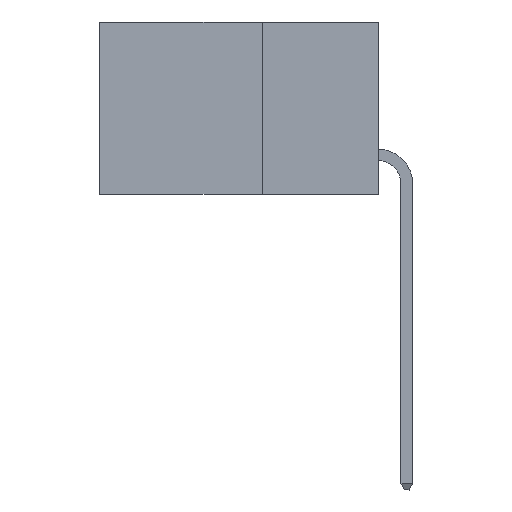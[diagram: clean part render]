
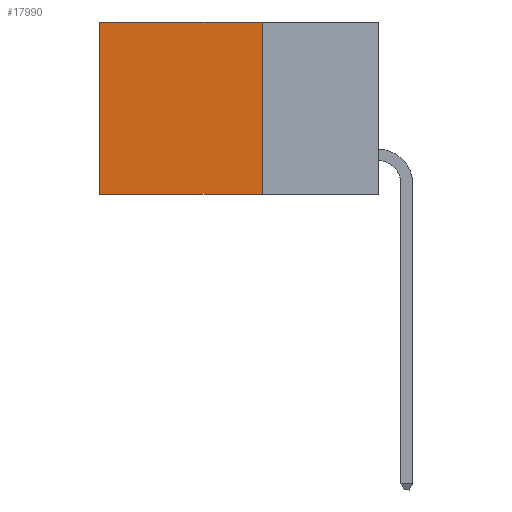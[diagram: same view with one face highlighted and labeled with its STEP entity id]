
A CAD part, left-side view. The second image highlights one B-rep face of the part: STEP entity #17990.
In plain terms, the highlighted planar face has unit normal (-1, 0, 0).
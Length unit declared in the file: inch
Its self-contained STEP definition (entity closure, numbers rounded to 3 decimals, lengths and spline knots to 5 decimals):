
#1260 = DIRECTION ( 'NONE',  ( 1., 0., 0. ) ) ;
#1993 = CARTESIAN_POINT ( 'NONE',  ( 0.298, 0.25, -0.37 ) ) ;
#3999 = LINE ( 'NONE', #11237, #13627 ) ;
#4737 = CARTESIAN_POINT ( 'NONE',  ( 0.298, 0.25, 0. ) ) ;
#4782 = VERTEX_POINT ( 'NONE', #7912 ) ;
#6050 = ORIENTED_EDGE ( 'NONE', *, *, #15029, .F. ) ;
#7912 = CARTESIAN_POINT ( 'NONE',  ( 0.298, 0.6, -0.37 ) ) ;
#7919 = CARTESIAN_POINT ( 'NONE',  ( 0.298, 0.6, 0. ) ) ;
#8032 = ORIENTED_EDGE ( 'NONE', *, *, #11321, .T. ) ;
#9610 = VECTOR ( 'NONE', #12752, 39.37008 ) ;
#9821 = VERTEX_POINT ( 'NONE', #23001 ) ;
#9860 = VECTOR ( 'NONE', #14388, 39.37008 ) ;
#10459 = LINE ( 'NONE', #4737, #9860 ) ;
#10761 = VECTOR ( 'NONE', #17360, 39.37008 ) ;
#11237 = CARTESIAN_POINT ( 'NONE',  ( 0.298, 0.6, 0. ) ) ;
#11321 = EDGE_CURVE ( 'NONE', #22218, #22830, #23883, .T. ) ;
#12752 = DIRECTION ( 'NONE',  ( 0., 1., 0. ) ) ;
#12774 = CARTESIAN_POINT ( 'NONE',  ( 0.298, 0.25, 0. ) ) ;
#13608 = FACE_OUTER_BOUND ( 'NONE', #23519, .T. ) ;
#13627 = VECTOR ( 'NONE', #18857, 39.37008 ) ;
#14388 = DIRECTION ( 'NONE',  ( 0., 0., -1. ) ) ;
#14480 = AXIS2_PLACEMENT_3D ( 'NONE', #12774, #1260, #14744 ) ;
#14744 = DIRECTION ( 'NONE',  ( 0., 0., -1. ) ) ;
#15029 = EDGE_CURVE ( 'NONE', #22218, #9821, #10459, .T. ) ;
#17271 = ORIENTED_EDGE ( 'NONE', *, *, #23285, .T. ) ;
#17360 = DIRECTION ( 'NONE',  ( 0., 1., 0. ) ) ;
#17990 = ADVANCED_FACE ( 'NONE', ( #13608 ), #23938, .F. ) ;
#18857 = DIRECTION ( 'NONE',  ( 0., 0., -1. ) ) ;
#19053 = ORIENTED_EDGE ( 'NONE', *, *, #21365, .F. ) ;
#21332 = LINE ( 'NONE', #1993, #10761 ) ;
#21365 = EDGE_CURVE ( 'NONE', #9821, #4782, #21332, .T. ) ;
#22218 = VERTEX_POINT ( 'NONE', #22613 ) ;
#22613 = CARTESIAN_POINT ( 'NONE',  ( 0.298, 0.25, 0. ) ) ;
#22830 = VERTEX_POINT ( 'NONE', #7919 ) ;
#23001 = CARTESIAN_POINT ( 'NONE',  ( 0.298, 0.25, -0.37 ) ) ;
#23285 = EDGE_CURVE ( 'NONE', #22830, #4782, #3999, .T. ) ;
#23519 = EDGE_LOOP ( 'NONE', ( #17271, #19053, #6050, #8032 ) ) ;
#23833 = CARTESIAN_POINT ( 'NONE',  ( 0.298, 0.25, 0. ) ) ;
#23883 = LINE ( 'NONE', #23833, #9610 ) ;
#23938 = PLANE ( 'NONE',  #14480 ) ;
